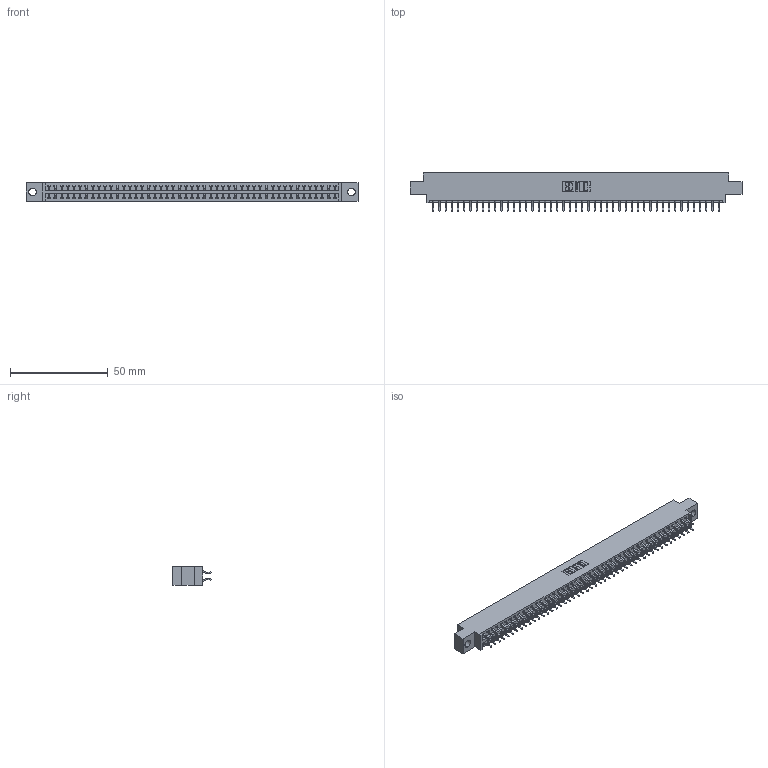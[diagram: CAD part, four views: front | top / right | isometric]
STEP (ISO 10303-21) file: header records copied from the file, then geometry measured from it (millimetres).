
FILE_DESCRIPTION (( 'STEP AP203' ), '1' );
FILE_NAME ('396-094-556-804.STEP', '2019-11-02T16:26:15', ( '' ), ( '' ), 'SwSTEP 2.0', 'SolidWorks 2016', '' );
FILE_SCHEMA (( 'CONFIG_CONTROL_DESIGN' ));
Length unit declared in the file: inch
Products named in the file (3): 346 Part_0.170 Offset - 0.156 Dia-TH; 345-292-001_556 Tail; 396-094-556-804
Assembly tree (95 placements, depth 2):
  396-094-556-804
    346 Part_0.170 Offset - 0.156 Dia-TH
    345-292-001_556 Tail  x94
Bounding box: 169.8 x 19.57 x 9.4 mm (x, y, z)
Volume: 16350.2 mm3; surface area: 22458.6 mm2
Topology: 95 solids, 95 shells, 5578 faces, 16603 edges, 10942 vertices
Faces by surface type: plane 3746, cylinder 1832
Entity records: 30355 total; most frequent: CARTESIAN_POINT 5012, ORIENTED_EDGE 4934, DIRECTION 4455, EDGE_CURVE 2467, LINE 2139, VECTOR 2139, VERTEX_POINT 1642, AXIS2_PLACEMENT_3D 1158
